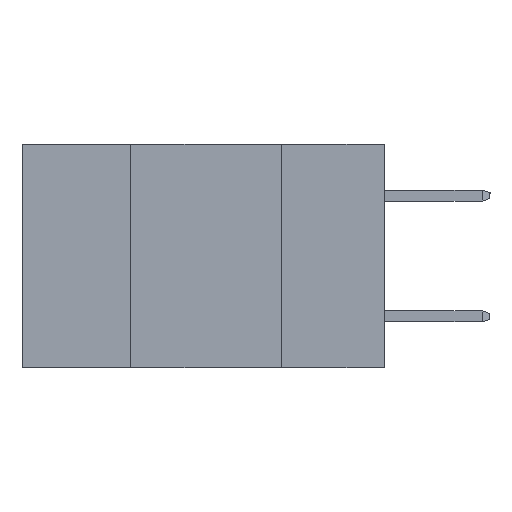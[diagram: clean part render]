
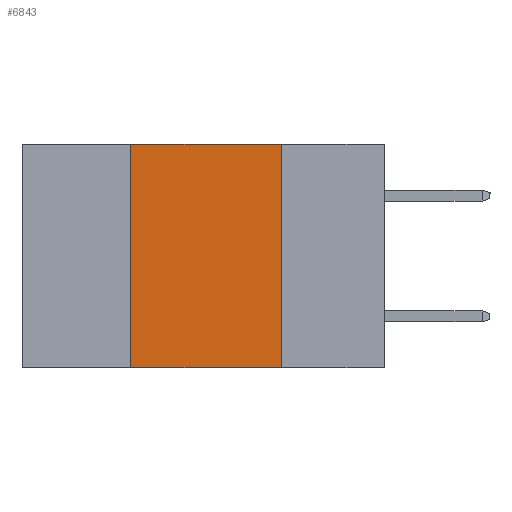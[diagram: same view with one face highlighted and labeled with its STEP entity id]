
A CAD part, left-side view. The second image highlights one B-rep face of the part: STEP entity #6843.
In plain terms, the highlighted planar face has unit normal (-1, 0, 0).
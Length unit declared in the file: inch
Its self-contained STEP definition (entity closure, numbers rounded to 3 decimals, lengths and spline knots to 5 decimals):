
#479 = CARTESIAN_POINT ( 'NONE',  ( 0., 0.6, -0.37 ) ) ;
#1584 = DIRECTION ( 'NONE',  ( 0., 0., -1. ) ) ;
#2345 = EDGE_CURVE ( 'NONE', #13126, #13162, #5448, .T. ) ;
#2430 = VECTOR ( 'NONE', #8288, 39.37008 ) ;
#2964 = PLANE ( 'NONE',  #10605 ) ;
#3401 = EDGE_CURVE ( 'NONE', #13162, #8871, #10726, .T. ) ;
#3402 = LINE ( 'NONE', #479, #9268 ) ;
#3958 = CARTESIAN_POINT ( 'NONE',  ( 0., 0.6, 0. ) ) ;
#4596 = DIRECTION ( 'NONE',  ( 0., 0., -1. ) ) ;
#4719 = EDGE_CURVE ( 'NONE', #8871, #7950, #16986, .T. ) ;
#5077 = ORIENTED_EDGE ( 'NONE', *, *, #13785, .T. ) ;
#5448 = LINE ( 'NONE', #10673, #2430 ) ;
#6537 = ORIENTED_EDGE ( 'NONE', *, *, #3401, .F. ) ;
#6843 = ADVANCED_FACE ( 'NONE', ( #10059 ), #2964, .F. ) ;
#7950 = VERTEX_POINT ( 'NONE', #15538 ) ;
#8154 = DIRECTION ( 'NONE',  ( 0., -1., 0. ) ) ;
#8288 = DIRECTION ( 'NONE',  ( 0., 0., 1. ) ) ;
#8522 = CARTESIAN_POINT ( 'NONE',  ( 0., 0.6, 0. ) ) ;
#8871 = VERTEX_POINT ( 'NONE', #12348 ) ;
#8880 = DIRECTION ( 'NONE',  ( 0., -1., 0. ) ) ;
#9268 = VECTOR ( 'NONE', #8880, 39.37008 ) ;
#9403 = EDGE_LOOP ( 'NONE', ( #15870, #6537, #9720, #5077 ) ) ;
#9720 = ORIENTED_EDGE ( 'NONE', *, *, #2345, .F. ) ;
#9976 = DIRECTION ( 'NONE',  ( 1., 0., 0. ) ) ;
#10059 = FACE_OUTER_BOUND ( 'NONE', #9403, .T. ) ;
#10605 = AXIS2_PLACEMENT_3D ( 'NONE', #8522, #9976, #1584 ) ;
#10673 = CARTESIAN_POINT ( 'NONE',  ( 0., 0.42, -0.37 ) ) ;
#10726 = LINE ( 'NONE', #3958, #12104 ) ;
#11960 = CARTESIAN_POINT ( 'NONE',  ( 0., 0.42, -0.37 ) ) ;
#12104 = VECTOR ( 'NONE', #8154, 39.37008 ) ;
#12348 = CARTESIAN_POINT ( 'NONE',  ( 0., 0.17, 0. ) ) ;
#12585 = CARTESIAN_POINT ( 'NONE',  ( 0., 0.42, 0. ) ) ;
#12632 = VECTOR ( 'NONE', #4596, 39.37008 ) ;
#13126 = VERTEX_POINT ( 'NONE', #11960 ) ;
#13162 = VERTEX_POINT ( 'NONE', #12585 ) ;
#13785 = EDGE_CURVE ( 'NONE', #13126, #7950, #3402, .T. ) ;
#14528 = CARTESIAN_POINT ( 'NONE',  ( 0., 0.17, -0.37 ) ) ;
#15538 = CARTESIAN_POINT ( 'NONE',  ( 0., 0.17, -0.37 ) ) ;
#15870 = ORIENTED_EDGE ( 'NONE', *, *, #4719, .F. ) ;
#16986 = LINE ( 'NONE', #14528, #12632 ) ;
